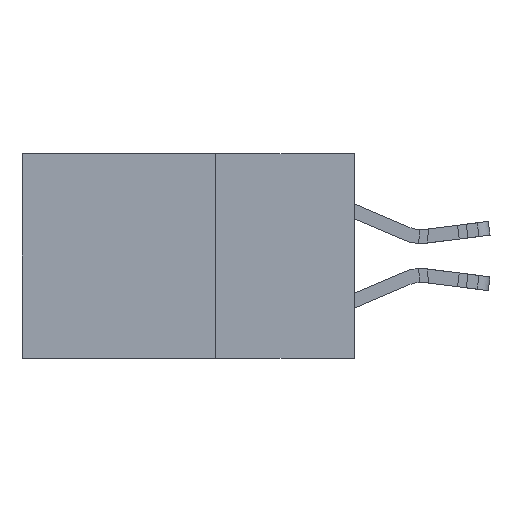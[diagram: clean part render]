
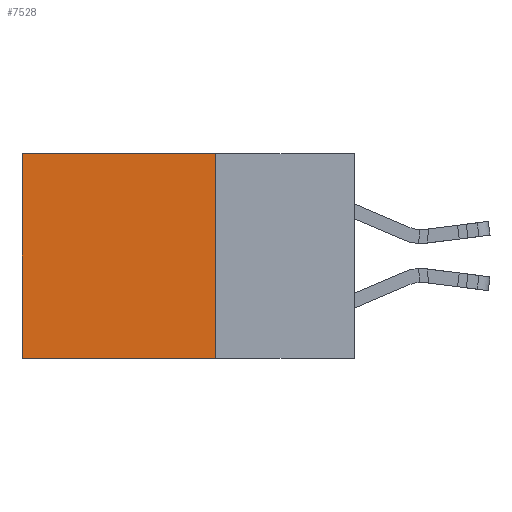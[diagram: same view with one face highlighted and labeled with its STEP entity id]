
A CAD part, left-side view. The second image highlights one B-rep face of the part: STEP entity #7528.
In plain terms, the highlighted planar face has unit normal (-1, 0, 0).
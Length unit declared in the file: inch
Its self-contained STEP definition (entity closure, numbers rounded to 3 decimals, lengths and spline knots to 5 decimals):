
#224 = EDGE_CURVE ( 'NONE', #15832, #11363, #13312, .T. ) ;
#525 = DIRECTION ( 'NONE',  ( 1., 0., 0. ) ) ;
#1311 = ORIENTED_EDGE ( 'NONE', *, *, #4836, .T. ) ;
#1555 = LINE ( 'NONE', #19320, #13212 ) ;
#3049 = DIRECTION ( 'NONE',  ( 0., 0., -1. ) ) ;
#3729 = LINE ( 'NONE', #18522, #15449 ) ;
#4401 = VECTOR ( 'NONE', #17326, 39.37008 ) ;
#4836 = EDGE_CURVE ( 'NONE', #15862, #15832, #3729, .T. ) ;
#6822 = DIRECTION ( 'NONE',  ( 0., 1., 0. ) ) ;
#6986 = CARTESIAN_POINT ( 'NONE',  ( 0.298, 0.25, 0. ) ) ;
#7528 = ADVANCED_FACE ( 'NONE', ( #18045 ), #12115, .F. ) ;
#9329 = EDGE_LOOP ( 'NONE', ( #20590, #20116, #14894, #1311 ) ) ;
#9593 = EDGE_CURVE ( 'NONE', #27710, #11363, #16858, .T. ) ;
#9849 = AXIS2_PLACEMENT_3D ( 'NONE', #28592, #525, #16878 ) ;
#11363 = VERTEX_POINT ( 'NONE', #24119 ) ;
#12115 = PLANE ( 'NONE',  #9849 ) ;
#13212 = VECTOR ( 'NONE', #3049, 39.37008 ) ;
#13312 = LINE ( 'NONE', #21548, #18822 ) ;
#13978 = CARTESIAN_POINT ( 'NONE',  ( 0.298, 0.6, 0. ) ) ;
#14894 = ORIENTED_EDGE ( 'NONE', *, *, #27061, .F. ) ;
#14983 = CARTESIAN_POINT ( 'NONE',  ( 0.298, 0.25, -0.37 ) ) ;
#15449 = VECTOR ( 'NONE', #6822, 39.37008 ) ;
#15832 = VERTEX_POINT ( 'NONE', #13978 ) ;
#15862 = VERTEX_POINT ( 'NONE', #6986 ) ;
#16858 = LINE ( 'NONE', #14983, #4401 ) ;
#16878 = DIRECTION ( 'NONE',  ( 0., 0., -1. ) ) ;
#17326 = DIRECTION ( 'NONE',  ( 0., 1., 0. ) ) ;
#18045 = FACE_OUTER_BOUND ( 'NONE', #9329, .T. ) ;
#18522 = CARTESIAN_POINT ( 'NONE',  ( 0.298, 0.25, 0. ) ) ;
#18822 = VECTOR ( 'NONE', #21580, 39.37008 ) ;
#19320 = CARTESIAN_POINT ( 'NONE',  ( 0.298, 0.25, 0. ) ) ;
#20116 = ORIENTED_EDGE ( 'NONE', *, *, #9593, .F. ) ;
#20590 = ORIENTED_EDGE ( 'NONE', *, *, #224, .T. ) ;
#21548 = CARTESIAN_POINT ( 'NONE',  ( 0.298, 0.6, 0. ) ) ;
#21580 = DIRECTION ( 'NONE',  ( 0., 0., -1. ) ) ;
#23501 = CARTESIAN_POINT ( 'NONE',  ( 0.298, 0.25, -0.37 ) ) ;
#24119 = CARTESIAN_POINT ( 'NONE',  ( 0.298, 0.6, -0.37 ) ) ;
#27061 = EDGE_CURVE ( 'NONE', #15862, #27710, #1555, .T. ) ;
#27710 = VERTEX_POINT ( 'NONE', #23501 ) ;
#28592 = CARTESIAN_POINT ( 'NONE',  ( 0.298, 0.25, 0. ) ) ;
